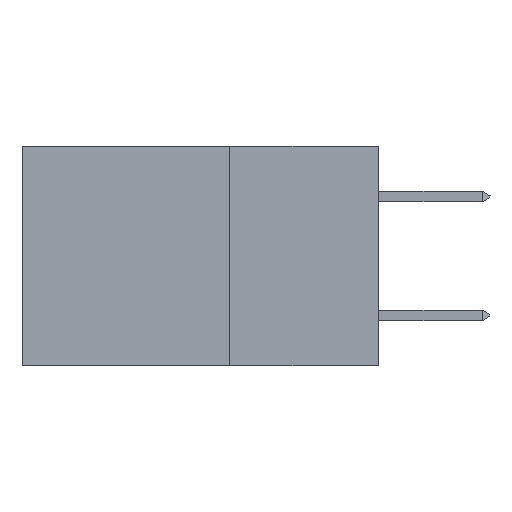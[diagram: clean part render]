
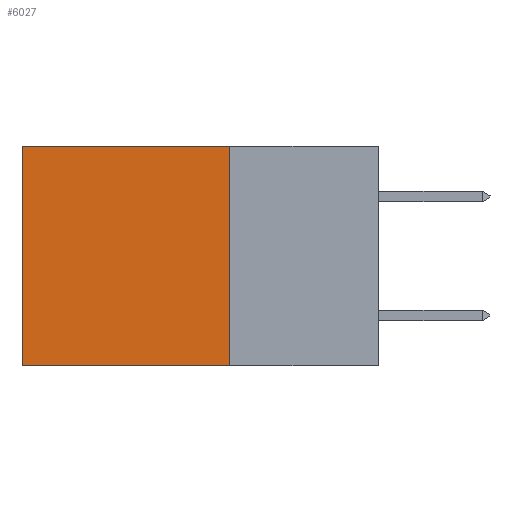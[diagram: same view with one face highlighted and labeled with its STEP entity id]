
A CAD part, left-side view. The second image highlights one B-rep face of the part: STEP entity #6027.
In plain terms, the highlighted planar face has unit normal (-1, 0, 0).
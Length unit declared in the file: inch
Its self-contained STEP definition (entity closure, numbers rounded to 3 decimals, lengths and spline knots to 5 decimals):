
#126 = CARTESIAN_POINT ( 'NONE',  ( 0.2615, 0.6, 0. ) ) ;
#164 = VERTEX_POINT ( 'NONE', #9212 ) ;
#904 = EDGE_LOOP ( 'NONE', ( #3008, #7898, #7966, #2502 ) ) ;
#942 = LINE ( 'NONE', #7865, #4704 ) ;
#969 = VECTOR ( 'NONE', #9375, 39.37008 ) ;
#2502 = ORIENTED_EDGE ( 'NONE', *, *, #8480, .T. ) ;
#2661 = PLANE ( 'NONE',  #7027 ) ;
#3002 = CARTESIAN_POINT ( 'NONE',  ( 0.2615, 0.25, 0. ) ) ;
#3008 = ORIENTED_EDGE ( 'NONE', *, *, #9687, .T. ) ;
#3232 = LINE ( 'NONE', #6270, #969 ) ;
#3263 = VECTOR ( 'NONE', #5311, 39.37008 ) ;
#3342 = DIRECTION ( 'NONE',  ( 0., 1., 0. ) ) ;
#3385 = CARTESIAN_POINT ( 'NONE',  ( 0.2615, 0.6, -0.37 ) ) ;
#3411 = FACE_OUTER_BOUND ( 'NONE', #904, .T. ) ;
#3760 = CARTESIAN_POINT ( 'NONE',  ( 0.2615, 0.25, -0.37 ) ) ;
#4087 = VECTOR ( 'NONE', #7306, 39.37008 ) ;
#4704 = VECTOR ( 'NONE', #3342, 39.37008 ) ;
#4938 = EDGE_CURVE ( 'NONE', #164, #6439, #3232, .T. ) ;
#4954 = DIRECTION ( 'NONE',  ( 0., 0., -1. ) ) ;
#5311 = DIRECTION ( 'NONE',  ( 0., 0., -1. ) ) ;
#5369 = LINE ( 'NONE', #8537, #3263 ) ;
#5709 = VERTEX_POINT ( 'NONE', #3002 ) ;
#5975 = LINE ( 'NONE', #3760, #4087 ) ;
#6027 = ADVANCED_FACE ( 'NONE', ( #3411 ), #2661, .F. ) ;
#6270 = CARTESIAN_POINT ( 'NONE',  ( 0.2615, 0.25, -0.37 ) ) ;
#6439 = VERTEX_POINT ( 'NONE', #3385 ) ;
#7027 = AXIS2_PLACEMENT_3D ( 'NONE', #8575, #8022, #4954 ) ;
#7306 = DIRECTION ( 'NONE',  ( 0., 0., -1. ) ) ;
#7796 = EDGE_CURVE ( 'NONE', #5709, #164, #5975, .T. ) ;
#7865 = CARTESIAN_POINT ( 'NONE',  ( 0.2615, 0.25, 0. ) ) ;
#7898 = ORIENTED_EDGE ( 'NONE', *, *, #4938, .F. ) ;
#7966 = ORIENTED_EDGE ( 'NONE', *, *, #7796, .F. ) ;
#8022 = DIRECTION ( 'NONE',  ( 1., 0., 0. ) ) ;
#8480 = EDGE_CURVE ( 'NONE', #5709, #8940, #942, .T. ) ;
#8537 = CARTESIAN_POINT ( 'NONE',  ( 0.2615, 0.6, -0.37 ) ) ;
#8575 = CARTESIAN_POINT ( 'NONE',  ( 0.2615, 0.25, -0.37 ) ) ;
#8940 = VERTEX_POINT ( 'NONE', #126 ) ;
#9212 = CARTESIAN_POINT ( 'NONE',  ( 0.2615, 0.25, -0.37 ) ) ;
#9375 = DIRECTION ( 'NONE',  ( 0., 1., 0. ) ) ;
#9687 = EDGE_CURVE ( 'NONE', #8940, #6439, #5369, .T. ) ;
